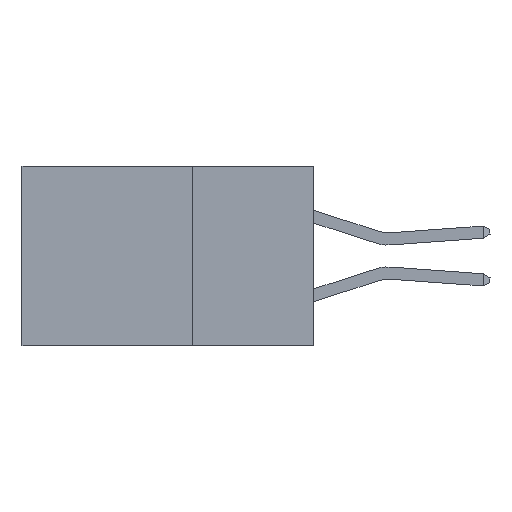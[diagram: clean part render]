
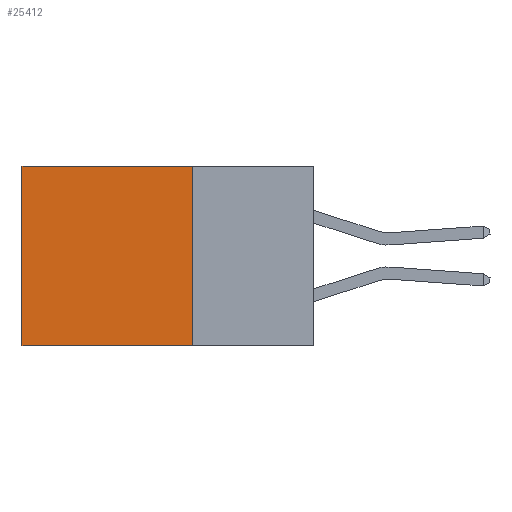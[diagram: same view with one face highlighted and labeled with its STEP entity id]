
A CAD part, left-side view. The second image highlights one B-rep face of the part: STEP entity #25412.
In plain terms, the highlighted planar face has unit normal (-1, 0, 0).
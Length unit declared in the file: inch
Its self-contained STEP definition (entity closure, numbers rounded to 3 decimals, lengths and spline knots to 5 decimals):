
#768 = VECTOR ( 'NONE', #27830, 39.37008 ) ;
#975 = EDGE_CURVE ( 'NONE', #25345, #36038, #23117, .T. ) ;
#2096 = PLANE ( 'NONE',  #21623 ) ;
#2247 = EDGE_CURVE ( 'NONE', #36038, #12542, #27920, .T. ) ;
#2975 = CARTESIAN_POINT ( 'NONE',  ( 0.2875, 0.25, -0.37 ) ) ;
#4869 = CARTESIAN_POINT ( 'NONE',  ( 0.2875, 0.6, 0. ) ) ;
#4940 = CARTESIAN_POINT ( 'NONE',  ( 0.2875, 0.25, 0. ) ) ;
#7322 = EDGE_CURVE ( 'NONE', #25345, #20427, #35461, .T. ) ;
#8604 = ORIENTED_EDGE ( 'NONE', *, *, #975, .T. ) ;
#9110 = DIRECTION ( 'NONE',  ( 0., 1., 0. ) ) ;
#9775 = ORIENTED_EDGE ( 'NONE', *, *, #2247, .T. ) ;
#12542 = VERTEX_POINT ( 'NONE', #34674 ) ;
#14361 = CARTESIAN_POINT ( 'NONE',  ( 0.2875, 0.6, 0. ) ) ;
#15006 = DIRECTION ( 'NONE',  ( 0., 0., -1. ) ) ;
#18171 = CARTESIAN_POINT ( 'NONE',  ( 0.2875, 0.25, 0. ) ) ;
#18670 = DIRECTION ( 'NONE',  ( 1., 0., 0. ) ) ;
#18946 = LINE ( 'NONE', #2975, #28997 ) ;
#20427 = VERTEX_POINT ( 'NONE', #24092 ) ;
#21623 = AXIS2_PLACEMENT_3D ( 'NONE', #4940, #18670, #29928 ) ;
#22215 = VECTOR ( 'NONE', #26808, 39.37008 ) ;
#23117 = LINE ( 'NONE', #35781, #768 ) ;
#23312 = CARTESIAN_POINT ( 'NONE',  ( 0.2875, 0.25, 0. ) ) ;
#24064 = EDGE_CURVE ( 'NONE', #20427, #12542, #18946, .T. ) ;
#24092 = CARTESIAN_POINT ( 'NONE',  ( 0.2875, 0.25, -0.37 ) ) ;
#25345 = VERTEX_POINT ( 'NONE', #18171 ) ;
#25412 = ADVANCED_FACE ( 'NONE', ( #31938 ), #2096, .F. ) ;
#26808 = DIRECTION ( 'NONE',  ( 0., 0., -1. ) ) ;
#27088 = ORIENTED_EDGE ( 'NONE', *, *, #7322, .F. ) ;
#27376 = EDGE_LOOP ( 'NONE', ( #9775, #33797, #27088, #8604 ) ) ;
#27830 = DIRECTION ( 'NONE',  ( 0., 1., 0. ) ) ;
#27920 = LINE ( 'NONE', #4869, #22215 ) ;
#28997 = VECTOR ( 'NONE', #9110, 39.37008 ) ;
#29928 = DIRECTION ( 'NONE',  ( 0., 0., -1. ) ) ;
#31495 = VECTOR ( 'NONE', #15006, 39.37008 ) ;
#31938 = FACE_OUTER_BOUND ( 'NONE', #27376, .T. ) ;
#33797 = ORIENTED_EDGE ( 'NONE', *, *, #24064, .F. ) ;
#34674 = CARTESIAN_POINT ( 'NONE',  ( 0.2875, 0.6, -0.37 ) ) ;
#35461 = LINE ( 'NONE', #23312, #31495 ) ;
#35781 = CARTESIAN_POINT ( 'NONE',  ( 0.2875, 0.25, 0. ) ) ;
#36038 = VERTEX_POINT ( 'NONE', #14361 ) ;
